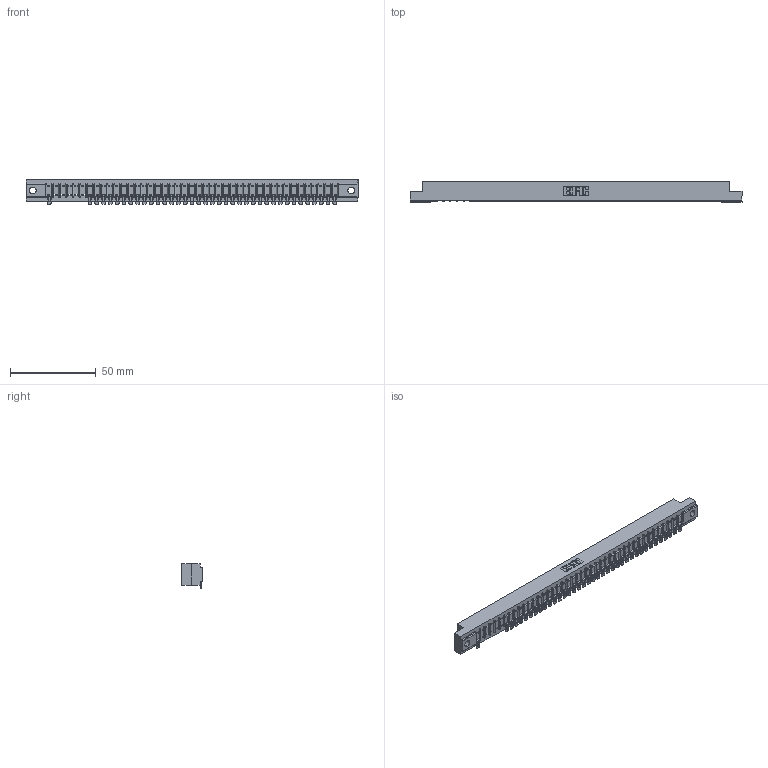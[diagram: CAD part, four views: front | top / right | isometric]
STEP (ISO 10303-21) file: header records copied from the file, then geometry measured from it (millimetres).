
FILE_DESCRIPTION (( 'STEP AP203' ), '1' );
FILE_NAME ('357-043-554-102.STEP', '2018-08-11T10:28:46', ( '' ), ( '' ), 'SwSTEP 2.0', 'SolidWorks 2016', '' );
FILE_SCHEMA (( 'CONFIG_CONTROL_DESIGN' ));
Length unit declared in the file: inch
Products named in the file (3): 307-290-002_554; 357-043-554-102; 307 Part_.128 Dia Mounting Holes
Assembly tree (39 placements, depth 2):
  357-043-554-102
    307 Part_.128 Dia Mounting Holes
    307-290-002_554  x38
Bounding box: 193.4 x 12.01 x 14.52 mm (x, y, z)
Volume: 20484.4 mm3; surface area: 24801 mm2
Topology: 39 solids, 39 shells, 3340 faces, 10257 edges, 6718 vertices
Faces by surface type: plane 1878, cylinder 1374, sphere 88
Entity records: 37547 total; most frequent: CARTESIAN_POINT 6357, ORIENTED_EDGE 6352, DIRECTION 6176, EDGE_CURVE 3176, LINE 2426, VECTOR 2426, VERTEX_POINT 2056, AXIS2_PLACEMENT_3D 1875
